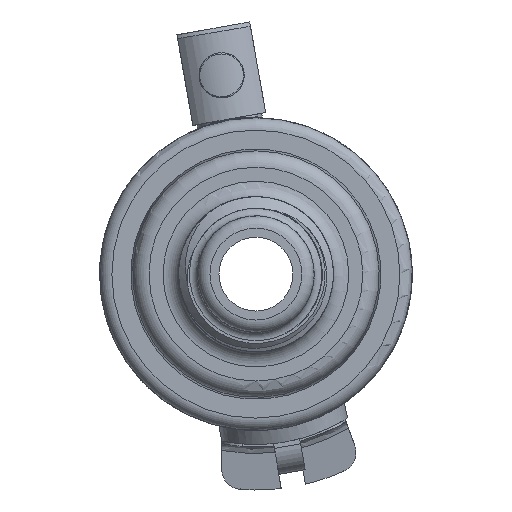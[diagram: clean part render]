
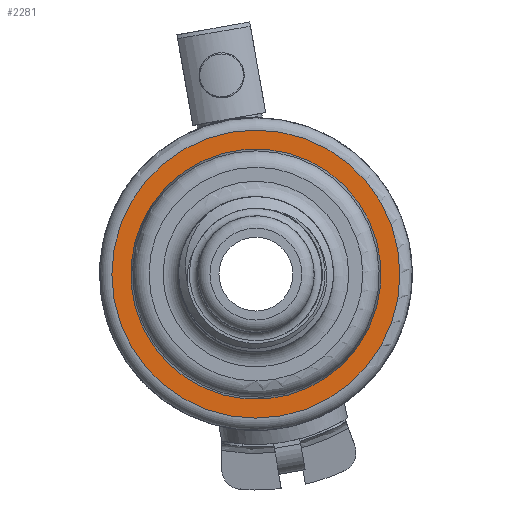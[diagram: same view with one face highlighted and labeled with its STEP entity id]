
A CAD part, left-side view. The second image highlights one B-rep face of the part: STEP entity #2281.
In plain terms, the highlighted planar face has unit normal (-1, 0, 0).
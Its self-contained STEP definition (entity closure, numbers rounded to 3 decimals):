
#55=FACE_BOUND('',#469,.T.);
#221=PLANE('',#2489);
#323=FACE_OUTER_BOUND('',#468,.T.);
#468=EDGE_LOOP('',(#1895));
#469=EDGE_LOOP('',(#1896));
#845=CIRCLE('',#2454,15.25);
#858=CIRCLE('',#2475,17.55);
#1012=VERTEX_POINT('',#8828);
#1021=VERTEX_POINT('',#8859);
#1300=EDGE_CURVE('',#1012,#1012,#845,.T.);
#1315=EDGE_CURVE('',#1021,#1021,#858,.T.);
#1895=ORIENTED_EDGE('',*,*,#1315,.F.);
#1896=ORIENTED_EDGE('',*,*,#1300,.T.);
#2281=ADVANCED_FACE('',(#323,#55),#221,.T.);
#2454=AXIS2_PLACEMENT_3D('',#8829,#2830,#2831);
#2475=AXIS2_PLACEMENT_3D('',#8861,#2874,#2875);
#2489=AXIS2_PLACEMENT_3D('',#9069,#2914,#2915);
#2830=DIRECTION('center_axis',(1.,0.,0.));
#2831=DIRECTION('ref_axis',(0.,-0.906,0.423));
#2874=DIRECTION('center_axis',(1.,0.,0.));
#2875=DIRECTION('ref_axis',(0.,-0.906,0.423));
#2914=DIRECTION('center_axis',(-1.,0.,0.));
#2915=DIRECTION('ref_axis',(0.,-0.985,0.174));
#8828=CARTESIAN_POINT('',(-84.5,13.821,-107.445));
#8829=CARTESIAN_POINT('Origin',(-84.5,0.,-101.));
#8859=CARTESIAN_POINT('',(-84.5,0.,-83.45));
#8861=CARTESIAN_POINT('Origin',(-84.5,0.,-101.));
#9069=CARTESIAN_POINT('Origin',(-84.5,0.017,-100.902));
